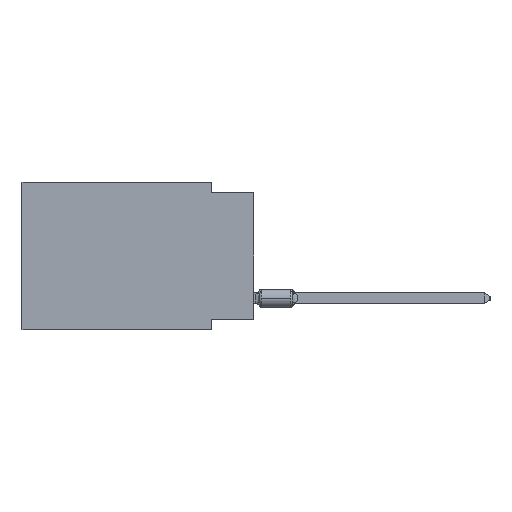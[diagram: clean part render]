
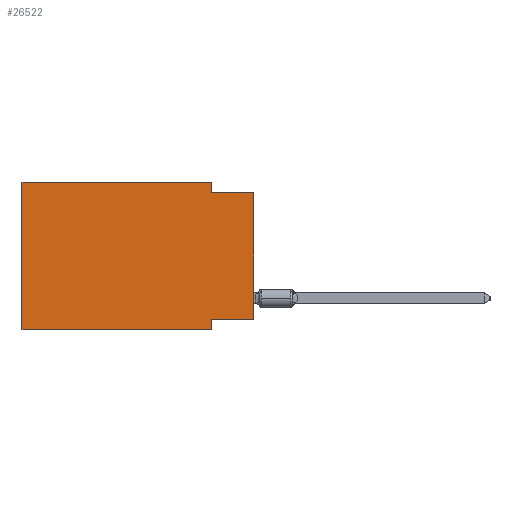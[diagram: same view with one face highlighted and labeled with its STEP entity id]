
A CAD part, left-side view. The second image highlights one B-rep face of the part: STEP entity #26522.
In plain terms, the highlighted planar face has unit normal (-1, 0, 0).
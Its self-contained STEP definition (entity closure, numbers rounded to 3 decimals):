
#3377 = CARTESIAN_POINT ( 'NONE',  ( 0., 2.54, 0. ) ) ;
#4890 = CARTESIAN_POINT ( 'NONE',  ( 0., 2.54, -8.89 ) ) ;
#7337 = CARTESIAN_POINT ( 'NONE',  ( 0., 13.97, 0. ) ) ;
#7972 = CARTESIAN_POINT ( 'NONE',  ( 0., 13.97, 0. ) ) ;
#9802 = CARTESIAN_POINT ( 'NONE',  ( 0., 13.97, -8.89 ) ) ;
#10059 = DIRECTION ( 'NONE',  ( 0., -1., 0. ) ) ;
#10665 = EDGE_CURVE ( 'NONE', #15412, #41513, #51808, .T. ) ;
#11199 = CARTESIAN_POINT ( 'NONE',  ( 0., 0., -0.635 ) ) ;
#11748 = VERTEX_POINT ( 'NONE', #3377 ) ;
#11842 = PLANE ( 'NONE',  #23003 ) ;
#12363 = EDGE_CURVE ( 'NONE', #46473, #49295, #40326, .T. ) ;
#12503 = ORIENTED_EDGE ( 'NONE', *, *, #12991, .T. ) ;
#12991 = EDGE_CURVE ( 'NONE', #15412, #49295, #50785, .T. ) ;
#13025 = VERTEX_POINT ( 'NONE', #19358 ) ;
#14542 = ORIENTED_EDGE ( 'NONE', *, *, #39347, .F. ) ;
#14999 = VECTOR ( 'NONE', #22780, 1000. ) ;
#15412 = VERTEX_POINT ( 'NONE', #52327 ) ;
#15451 = VECTOR ( 'NONE', #10059, 1000. ) ;
#15830 = FACE_OUTER_BOUND ( 'NONE', #23093, .T. ) ;
#17430 = EDGE_CURVE ( 'NONE', #39284, #31619, #20253, .T. ) ;
#18149 = VECTOR ( 'NONE', #34509, 1000. ) ;
#19358 = CARTESIAN_POINT ( 'NONE',  ( 0., 0., -8.255 ) ) ;
#19429 = CARTESIAN_POINT ( 'NONE',  ( 0., 2.54, -0.635 ) ) ;
#19525 = CARTESIAN_POINT ( 'NONE',  ( 0., 2.54, -8.255 ) ) ;
#20077 = DIRECTION ( 'NONE',  ( 0., 0., -1. ) ) ;
#20253 = LINE ( 'NONE', #11199, #31953 ) ;
#20315 = CARTESIAN_POINT ( 'NONE',  ( 0., 0., -0.635 ) ) ;
#20344 = DIRECTION ( 'NONE',  ( 1., 0., 0. ) ) ;
#20485 = DIRECTION ( 'NONE',  ( 0., -1., 0. ) ) ;
#22203 = CARTESIAN_POINT ( 'NONE',  ( 0., 13.97, 0. ) ) ;
#22780 = DIRECTION ( 'NONE',  ( 0., 0., -1. ) ) ;
#23003 = AXIS2_PLACEMENT_3D ( 'NONE', #45099, #20344, #24603 ) ;
#23093 = EDGE_LOOP ( 'NONE', ( #25476, #28740, #37912, #14542, #30158, #12503, #49816, #52492 ) ) ;
#24603 = DIRECTION ( 'NONE',  ( 0., 0., -1. ) ) ;
#25264 = LINE ( 'NONE', #7972, #50294 ) ;
#25476 = ORIENTED_EDGE ( 'NONE', *, *, #31044, .T. ) ;
#25726 = LINE ( 'NONE', #35459, #29299 ) ;
#26010 = CARTESIAN_POINT ( 'NONE',  ( 0., 0., 0. ) ) ;
#26522 = ADVANCED_FACE ( 'NONE', ( #15830 ), #11842, .F. ) ;
#28740 = ORIENTED_EDGE ( 'NONE', *, *, #17430, .F. ) ;
#28819 = LINE ( 'NONE', #39771, #14999 ) ;
#29023 = VECTOR ( 'NONE', #20077, 1000. ) ;
#29299 = VECTOR ( 'NONE', #37699, 1000. ) ;
#30158 = ORIENTED_EDGE ( 'NONE', *, *, #10665, .F. ) ;
#31044 = EDGE_CURVE ( 'NONE', #13025, #31619, #38517, .T. ) ;
#31619 = VERTEX_POINT ( 'NONE', #20315 ) ;
#31953 = VECTOR ( 'NONE', #31971, 1000. ) ;
#31971 = DIRECTION ( 'NONE',  ( 0., -1., 0. ) ) ;
#32776 = CARTESIAN_POINT ( 'NONE',  ( 0., 2.54, -8.89 ) ) ;
#34509 = DIRECTION ( 'NONE',  ( 0., 0., 1. ) ) ;
#35459 = CARTESIAN_POINT ( 'NONE',  ( 0., 0., -8.255 ) ) ;
#37699 = DIRECTION ( 'NONE',  ( 0., 1., 0. ) ) ;
#37912 = ORIENTED_EDGE ( 'NONE', *, *, #46411, .F. ) ;
#38517 = LINE ( 'NONE', #26010, #18149 ) ;
#39284 = VERTEX_POINT ( 'NONE', #19429 ) ;
#39347 = EDGE_CURVE ( 'NONE', #41513, #11748, #25264, .T. ) ;
#39771 = CARTESIAN_POINT ( 'NONE',  ( 0., 2.54, 0. ) ) ;
#40326 = LINE ( 'NONE', #4890, #29023 ) ;
#41513 = VERTEX_POINT ( 'NONE', #22203 ) ;
#45099 = CARTESIAN_POINT ( 'NONE',  ( 0., 13.97, 0. ) ) ;
#46411 = EDGE_CURVE ( 'NONE', #11748, #39284, #28819, .T. ) ;
#46473 = VERTEX_POINT ( 'NONE', #19525 ) ;
#48331 = DIRECTION ( 'NONE',  ( 0., 0., 1. ) ) ;
#49295 = VERTEX_POINT ( 'NONE', #32776 ) ;
#49816 = ORIENTED_EDGE ( 'NONE', *, *, #12363, .F. ) ;
#50264 = EDGE_CURVE ( 'NONE', #13025, #46473, #25726, .T. ) ;
#50294 = VECTOR ( 'NONE', #20485, 1000. ) ;
#50785 = LINE ( 'NONE', #9802, #15451 ) ;
#51004 = VECTOR ( 'NONE', #48331, 1000. ) ;
#51808 = LINE ( 'NONE', #7337, #51004 ) ;
#52327 = CARTESIAN_POINT ( 'NONE',  ( 0., 13.97, -8.89 ) ) ;
#52492 = ORIENTED_EDGE ( 'NONE', *, *, #50264, .F. ) ;
